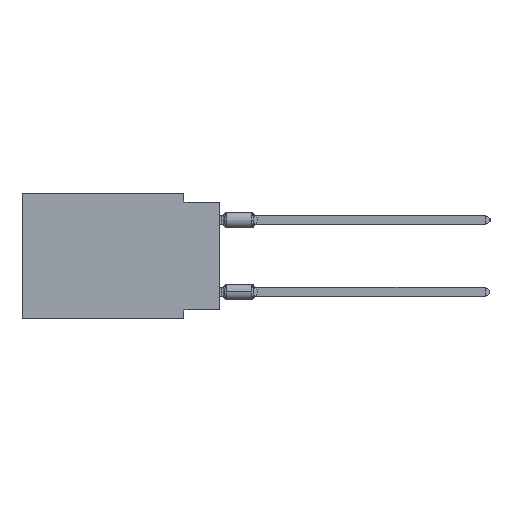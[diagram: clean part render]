
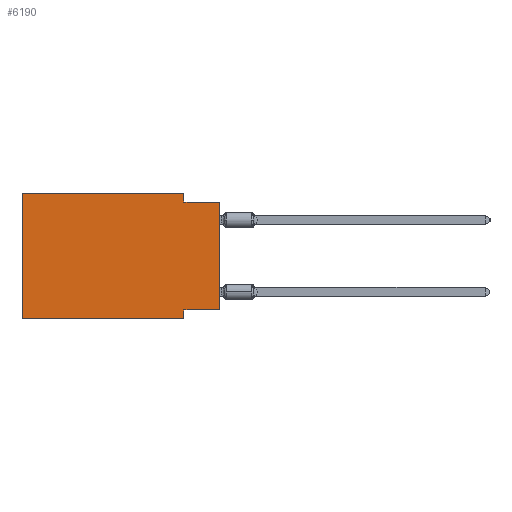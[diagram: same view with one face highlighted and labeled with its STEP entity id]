
A CAD part, left-side view. The second image highlights one B-rep face of the part: STEP entity #6190.
In plain terms, the highlighted planar face has unit normal (-1, 0, 0).
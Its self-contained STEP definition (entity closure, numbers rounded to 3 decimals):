
#235 = DIRECTION ( 'NONE',  ( 0., -1., 0. ) ) ;
#1071 = EDGE_CURVE ( 'NONE', #37237, #28347, #8583, .T. ) ;
#1977 = VERTEX_POINT ( 'NONE', #32604 ) ;
#2437 = VECTOR ( 'NONE', #18527, 1000. ) ;
#2738 = ORIENTED_EDGE ( 'NONE', *, *, #35482, .F. ) ;
#2753 = CARTESIAN_POINT ( 'NONE',  ( 0., 0., -0.635 ) ) ;
#4427 = CARTESIAN_POINT ( 'NONE',  ( 0., 13.97, -8.89 ) ) ;
#4796 = VECTOR ( 'NONE', #11454, 1000. ) ;
#4862 = CARTESIAN_POINT ( 'NONE',  ( 0., 2.54, -8.89 ) ) ;
#5235 = VECTOR ( 'NONE', #31664, 1000. ) ;
#6190 = ADVANCED_FACE ( 'NONE', ( #9681 ), #35764, .F. ) ;
#8013 = DIRECTION ( 'NONE',  ( 0., 0., 1. ) ) ;
#8113 = LINE ( 'NONE', #19892, #5235 ) ;
#8168 = CARTESIAN_POINT ( 'NONE',  ( 0., 2.54, -8.89 ) ) ;
#8583 = LINE ( 'NONE', #29064, #13207 ) ;
#9072 = VERTEX_POINT ( 'NONE', #27535 ) ;
#9112 = CARTESIAN_POINT ( 'NONE',  ( 0., 13.97, 0. ) ) ;
#9558 = CARTESIAN_POINT ( 'NONE',  ( 0., 2.54, 0. ) ) ;
#9681 = FACE_OUTER_BOUND ( 'NONE', #23284, .T. ) ;
#11454 = DIRECTION ( 'NONE',  ( 0., 0., -1. ) ) ;
#12042 = LINE ( 'NONE', #2753, #12364 ) ;
#12364 = VECTOR ( 'NONE', #235, 1000. ) ;
#12456 = ORIENTED_EDGE ( 'NONE', *, *, #24242, .F. ) ;
#12626 = EDGE_CURVE ( 'NONE', #1977, #22427, #30012, .T. ) ;
#13207 = VECTOR ( 'NONE', #8013, 1000. ) ;
#13395 = ORIENTED_EDGE ( 'NONE', *, *, #13545, .T. ) ;
#13545 = EDGE_CURVE ( 'NONE', #1977, #37866, #24876, .T. ) ;
#13586 = ORIENTED_EDGE ( 'NONE', *, *, #25704, .F. ) ;
#13823 = ORIENTED_EDGE ( 'NONE', *, *, #1071, .F. ) ;
#14065 = VECTOR ( 'NONE', #24420, 1000. ) ;
#15522 = DIRECTION ( 'NONE',  ( 0., 1., 0. ) ) ;
#15540 = LINE ( 'NONE', #9558, #14065 ) ;
#15548 = VECTOR ( 'NONE', #38117, 1000. ) ;
#18527 = DIRECTION ( 'NONE',  ( 0., 0., 1. ) ) ;
#18904 = CARTESIAN_POINT ( 'NONE',  ( 0., 0., 0. ) ) ;
#18931 = AXIS2_PLACEMENT_3D ( 'NONE', #9112, #27257, #20887 ) ;
#19497 = CARTESIAN_POINT ( 'NONE',  ( 0., 2.54, -0.635 ) ) ;
#19892 = CARTESIAN_POINT ( 'NONE',  ( 0., 13.97, -8.89 ) ) ;
#20887 = DIRECTION ( 'NONE',  ( 0., 0., -1. ) ) ;
#21310 = CARTESIAN_POINT ( 'NONE',  ( 0., 0., -8.255 ) ) ;
#22427 = VERTEX_POINT ( 'NONE', #30847 ) ;
#23058 = CARTESIAN_POINT ( 'NONE',  ( 0., 13.97, 0. ) ) ;
#23284 = EDGE_LOOP ( 'NONE', ( #13395, #2738, #12456, #13586, #13823, #30785, #37720, #33202 ) ) ;
#23982 = VECTOR ( 'NONE', #15522, 1000. ) ;
#24242 = EDGE_CURVE ( 'NONE', #9072, #26431, #15540, .T. ) ;
#24420 = DIRECTION ( 'NONE',  ( 0., 0., -1. ) ) ;
#24876 = LINE ( 'NONE', #18904, #2437 ) ;
#25704 = EDGE_CURVE ( 'NONE', #28347, #9072, #34642, .T. ) ;
#26431 = VERTEX_POINT ( 'NONE', #19497 ) ;
#27257 = DIRECTION ( 'NONE',  ( 1., 0., 0. ) ) ;
#27535 = CARTESIAN_POINT ( 'NONE',  ( 0., 2.54, 0. ) ) ;
#28246 = VERTEX_POINT ( 'NONE', #4862 ) ;
#28347 = VERTEX_POINT ( 'NONE', #34607 ) ;
#29064 = CARTESIAN_POINT ( 'NONE',  ( 0., 13.97, 0. ) ) ;
#30012 = LINE ( 'NONE', #21310, #23982 ) ;
#30702 = EDGE_CURVE ( 'NONE', #22427, #28246, #37716, .T. ) ;
#30785 = ORIENTED_EDGE ( 'NONE', *, *, #37467, .T. ) ;
#30847 = CARTESIAN_POINT ( 'NONE',  ( 0., 2.54, -8.255 ) ) ;
#31664 = DIRECTION ( 'NONE',  ( 0., -1., 0. ) ) ;
#32604 = CARTESIAN_POINT ( 'NONE',  ( 0., 0., -8.255 ) ) ;
#33202 = ORIENTED_EDGE ( 'NONE', *, *, #12626, .F. ) ;
#34607 = CARTESIAN_POINT ( 'NONE',  ( 0., 13.97, 0. ) ) ;
#34642 = LINE ( 'NONE', #23058, #15548 ) ;
#35482 = EDGE_CURVE ( 'NONE', #26431, #37866, #12042, .T. ) ;
#35764 = PLANE ( 'NONE',  #18931 ) ;
#37227 = CARTESIAN_POINT ( 'NONE',  ( 0., 0., -0.635 ) ) ;
#37237 = VERTEX_POINT ( 'NONE', #4427 ) ;
#37467 = EDGE_CURVE ( 'NONE', #37237, #28246, #8113, .T. ) ;
#37716 = LINE ( 'NONE', #8168, #4796 ) ;
#37720 = ORIENTED_EDGE ( 'NONE', *, *, #30702, .F. ) ;
#37866 = VERTEX_POINT ( 'NONE', #37227 ) ;
#38117 = DIRECTION ( 'NONE',  ( 0., -1., 0. ) ) ;
